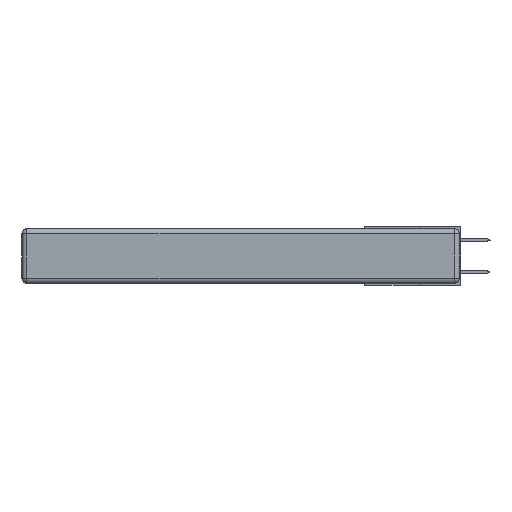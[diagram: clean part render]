
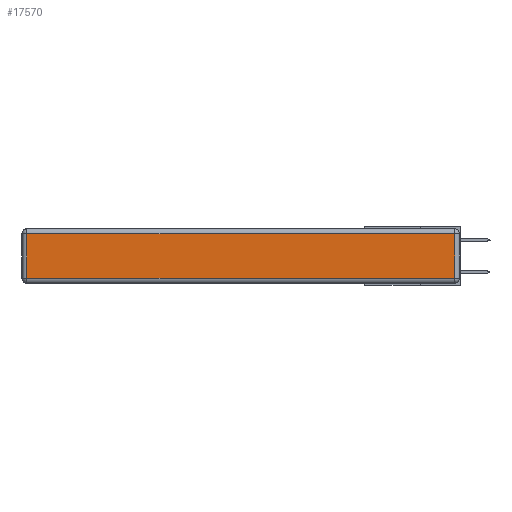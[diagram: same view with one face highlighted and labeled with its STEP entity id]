
A CAD part, left-side view. The second image highlights one B-rep face of the part: STEP entity #17570.
In plain terms, the highlighted planar face has unit normal (-1, 0, 0).
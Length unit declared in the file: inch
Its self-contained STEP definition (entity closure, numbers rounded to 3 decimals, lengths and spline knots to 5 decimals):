
#205 = CARTESIAN_POINT ( 'NONE',  ( 0., 2.72, -0.343 ) ) ;
#1613 = CARTESIAN_POINT ( 'NONE',  ( 0., 2.75, -0.03 ) ) ;
#1631 = VERTEX_POINT ( 'NONE', #7991 ) ;
#2094 = EDGE_CURVE ( 'NONE', #2599, #1631, #3540, .T. ) ;
#2599 = VERTEX_POINT ( 'NONE', #2868 ) ;
#2868 = CARTESIAN_POINT ( 'NONE',  ( 0., 0.03, -0.03 ) ) ;
#2888 = LINE ( 'NONE', #7043, #13730 ) ;
#3540 = LINE ( 'NONE', #1613, #6426 ) ;
#4847 = DIRECTION ( 'NONE',  ( 0., 1., 0. ) ) ;
#4908 = ORIENTED_EDGE ( 'NONE', *, *, #14660, .T. ) ;
#5209 = DIRECTION ( 'NONE',  ( 0., 0., -1. ) ) ;
#5947 = ORIENTED_EDGE ( 'NONE', *, *, #2094, .T. ) ;
#6407 = EDGE_LOOP ( 'NONE', ( #18486, #6813, #5947, #4908 ) ) ;
#6426 = VECTOR ( 'NONE', #4847, 39.37008 ) ;
#6438 = EDGE_CURVE ( 'NONE', #17087, #12914, #16145, .T. ) ;
#6666 = VECTOR ( 'NONE', #5209, 39.37008 ) ;
#6813 = ORIENTED_EDGE ( 'NONE', *, *, #16538, .T. ) ;
#7043 = CARTESIAN_POINT ( 'NONE',  ( 0., 0.03, -0.343 ) ) ;
#7991 = CARTESIAN_POINT ( 'NONE',  ( 0., 2.72, -0.03 ) ) ;
#8530 = LINE ( 'NONE', #205, #6666 ) ;
#8790 = DIRECTION ( 'NONE',  ( -1., 0., 0. ) ) ;
#10808 = CARTESIAN_POINT ( 'NONE',  ( 0., 0.03, -0.313 ) ) ;
#11051 = AXIS2_PLACEMENT_3D ( 'NONE', #12051, #8790, #15288 ) ;
#11679 = VECTOR ( 'NONE', #12121, 39.37008 ) ;
#12051 = CARTESIAN_POINT ( 'NONE',  ( 0., 0., -0.343 ) ) ;
#12121 = DIRECTION ( 'NONE',  ( 0., -1., 0. ) ) ;
#12914 = VERTEX_POINT ( 'NONE', #10808 ) ;
#13730 = VECTOR ( 'NONE', #13941, 39.37008 ) ;
#13941 = DIRECTION ( 'NONE',  ( 0., 0., 1. ) ) ;
#14660 = EDGE_CURVE ( 'NONE', #1631, #17087, #8530, .T. ) ;
#15274 = FACE_OUTER_BOUND ( 'NONE', #6407, .T. ) ;
#15288 = DIRECTION ( 'NONE',  ( 0., 0., 1. ) ) ;
#15498 = PLANE ( 'NONE',  #11051 ) ;
#16145 = LINE ( 'NONE', #18977, #11679 ) ;
#16538 = EDGE_CURVE ( 'NONE', #12914, #2599, #2888, .T. ) ;
#17087 = VERTEX_POINT ( 'NONE', #18858 ) ;
#17570 = ADVANCED_FACE ( 'NONE', ( #15274 ), #15498, .T. ) ;
#18486 = ORIENTED_EDGE ( 'NONE', *, *, #6438, .T. ) ;
#18858 = CARTESIAN_POINT ( 'NONE',  ( 0., 2.72, -0.313 ) ) ;
#18977 = CARTESIAN_POINT ( 'NONE',  ( 0., 0., -0.313 ) ) ;
